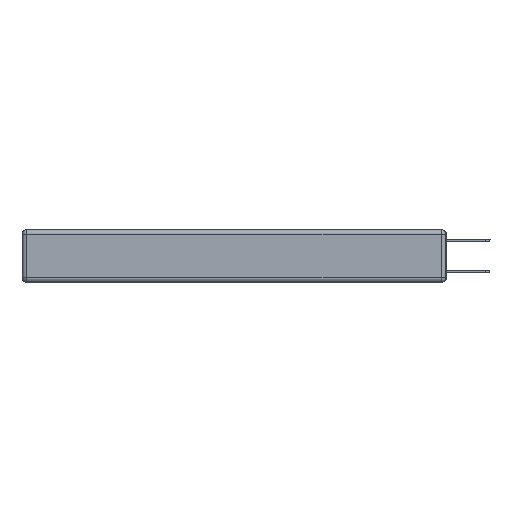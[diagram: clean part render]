
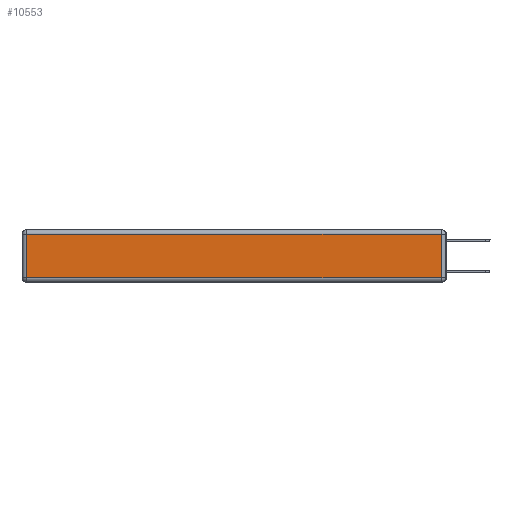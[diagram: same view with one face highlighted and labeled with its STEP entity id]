
A CAD part, left-side view. The second image highlights one B-rep face of the part: STEP entity #10553.
In plain terms, the highlighted planar face has unit normal (-1, 0, 0).
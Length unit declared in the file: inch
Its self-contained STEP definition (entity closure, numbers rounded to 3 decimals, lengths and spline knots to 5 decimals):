
#30 = LINE ( 'NONE', #19231, #25415 ) ;
#36 = CARTESIAN_POINT ( 'NONE',  ( 0., 0.03, -0.03 ) ) ;
#178 = EDGE_CURVE ( 'NONE', #2405, #8948, #6228, .T. ) ;
#819 = DIRECTION ( 'NONE',  ( 0., -1., 0. ) ) ;
#833 = EDGE_CURVE ( 'NONE', #15760, #8107, #30, .T. ) ;
#1043 = LINE ( 'NONE', #20492, #8978 ) ;
#1439 = CARTESIAN_POINT ( 'NONE',  ( 0., 2.72, -0.03 ) ) ;
#1626 = PLANE ( 'NONE',  #2658 ) ;
#2237 = EDGE_LOOP ( 'NONE', ( #23705, #6738, #26057, #10886 ) ) ;
#2405 = VERTEX_POINT ( 'NONE', #36 ) ;
#2658 = AXIS2_PLACEMENT_3D ( 'NONE', #10234, #5688, #12209 ) ;
#5652 = DIRECTION ( 'NONE',  ( 0., 0., -1. ) ) ;
#5688 = DIRECTION ( 'NONE',  ( -1., 0., 0. ) ) ;
#6228 = LINE ( 'NONE', #8907, #24065 ) ;
#6738 = ORIENTED_EDGE ( 'NONE', *, *, #12395, .T. ) ;
#8107 = VERTEX_POINT ( 'NONE', #22827 ) ;
#8213 = DIRECTION ( 'NONE',  ( 0., 0., 1. ) ) ;
#8447 = VECTOR ( 'NONE', #8213, 39.37008 ) ;
#8907 = CARTESIAN_POINT ( 'NONE',  ( 0., 2.75, -0.03 ) ) ;
#8948 = VERTEX_POINT ( 'NONE', #1439 ) ;
#8978 = VECTOR ( 'NONE', #5652, 39.37008 ) ;
#10234 = CARTESIAN_POINT ( 'NONE',  ( 0., 0., -0.343 ) ) ;
#10553 = ADVANCED_FACE ( 'NONE', ( #24997 ), #1626, .T. ) ;
#10886 = ORIENTED_EDGE ( 'NONE', *, *, #11023, .T. ) ;
#11023 = EDGE_CURVE ( 'NONE', #8948, #15760, #1043, .T. ) ;
#12209 = DIRECTION ( 'NONE',  ( 0., 0., 1. ) ) ;
#12395 = EDGE_CURVE ( 'NONE', #8107, #2405, #17106, .T. ) ;
#15760 = VERTEX_POINT ( 'NONE', #21276 ) ;
#17106 = LINE ( 'NONE', #23717, #8447 ) ;
#19231 = CARTESIAN_POINT ( 'NONE',  ( 0., 0., -0.313 ) ) ;
#20492 = CARTESIAN_POINT ( 'NONE',  ( 0., 2.72, -0.343 ) ) ;
#21276 = CARTESIAN_POINT ( 'NONE',  ( 0., 2.72, -0.313 ) ) ;
#22827 = CARTESIAN_POINT ( 'NONE',  ( 0., 0.03, -0.313 ) ) ;
#23705 = ORIENTED_EDGE ( 'NONE', *, *, #833, .T. ) ;
#23717 = CARTESIAN_POINT ( 'NONE',  ( 0., 0.03, -0.343 ) ) ;
#24065 = VECTOR ( 'NONE', #27797, 39.37008 ) ;
#24997 = FACE_OUTER_BOUND ( 'NONE', #2237, .T. ) ;
#25415 = VECTOR ( 'NONE', #819, 39.37008 ) ;
#26057 = ORIENTED_EDGE ( 'NONE', *, *, #178, .T. ) ;
#27797 = DIRECTION ( 'NONE',  ( 0., 1., 0. ) ) ;
